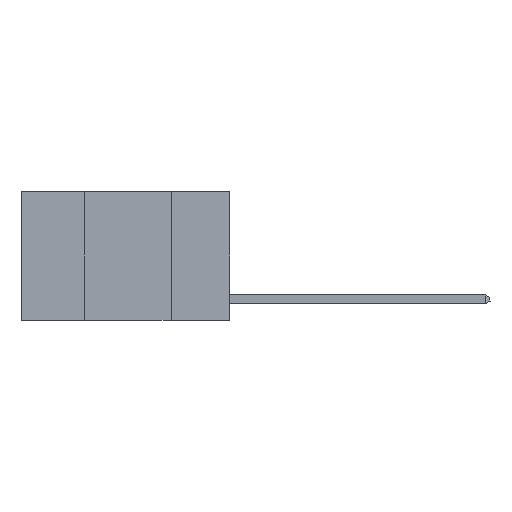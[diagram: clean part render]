
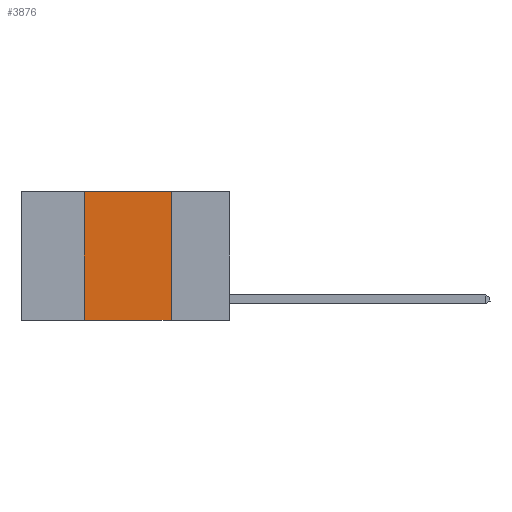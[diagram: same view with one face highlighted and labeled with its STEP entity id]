
A CAD part, left-side view. The second image highlights one B-rep face of the part: STEP entity #3876.
In plain terms, the highlighted planar face has unit normal (-1, 0, 0).
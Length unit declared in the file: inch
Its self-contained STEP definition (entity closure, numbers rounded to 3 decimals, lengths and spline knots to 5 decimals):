
#1446 = EDGE_CURVE ( 'NONE', #4142, #4504, #2782, .T. ) ;
#2782 = LINE ( 'NONE', #12712, #23775 ) ;
#3180 = AXIS2_PLACEMENT_3D ( 'NONE', #5985, #12367, #26948 ) ;
#3876 = ADVANCED_FACE ( 'NONE', ( #21820 ), #16523, .F. ) ;
#4142 = VERTEX_POINT ( 'NONE', #23662 ) ;
#4504 = VERTEX_POINT ( 'NONE', #22647 ) ;
#5744 = VECTOR ( 'NONE', #5981, 39.37008 ) ;
#5981 = DIRECTION ( 'NONE',  ( 0., -1., 0. ) ) ;
#5985 = CARTESIAN_POINT ( 'NONE',  ( 0., 0.6, 0. ) ) ;
#6893 = EDGE_CURVE ( 'NONE', #4504, #24385, #7233, .T. ) ;
#7233 = LINE ( 'NONE', #17156, #17783 ) ;
#7888 = CARTESIAN_POINT ( 'NONE',  ( 0., 0.17, -0.37 ) ) ;
#8192 = ORIENTED_EDGE ( 'NONE', *, *, #23771, .T. ) ;
#10487 = DIRECTION ( 'NONE',  ( 0., -1., 0. ) ) ;
#11844 = ORIENTED_EDGE ( 'NONE', *, *, #1446, .F. ) ;
#12367 = DIRECTION ( 'NONE',  ( 1., 0., 0. ) ) ;
#12712 = CARTESIAN_POINT ( 'NONE',  ( 0., 0.6, 0. ) ) ;
#14300 = CARTESIAN_POINT ( 'NONE',  ( 0., 0.42, 0. ) ) ;
#15680 = EDGE_CURVE ( 'NONE', #21870, #4142, #24409, .T. ) ;
#16521 = CARTESIAN_POINT ( 'NONE',  ( 0., 0.6, -0.37 ) ) ;
#16523 = PLANE ( 'NONE',  #3180 ) ;
#17156 = CARTESIAN_POINT ( 'NONE',  ( 0., 0.17, 0. ) ) ;
#17783 = VECTOR ( 'NONE', #19233, 39.37008 ) ;
#18492 = DIRECTION ( 'NONE',  ( 0., 0., 1. ) ) ;
#19233 = DIRECTION ( 'NONE',  ( 0., 0., -1. ) ) ;
#20219 = CARTESIAN_POINT ( 'NONE',  ( 0., 0.42, -0.37 ) ) ;
#21820 = FACE_OUTER_BOUND ( 'NONE', #22586, .T. ) ;
#21870 = VERTEX_POINT ( 'NONE', #20219 ) ;
#22305 = ORIENTED_EDGE ( 'NONE', *, *, #6893, .F. ) ;
#22486 = LINE ( 'NONE', #16521, #5744 ) ;
#22586 = EDGE_LOOP ( 'NONE', ( #22305, #11844, #24246, #8192 ) ) ;
#22647 = CARTESIAN_POINT ( 'NONE',  ( 0., 0.17, 0. ) ) ;
#23662 = CARTESIAN_POINT ( 'NONE',  ( 0., 0.42, 0. ) ) ;
#23771 = EDGE_CURVE ( 'NONE', #21870, #24385, #22486, .T. ) ;
#23775 = VECTOR ( 'NONE', #10487, 39.37008 ) ;
#23777 = VECTOR ( 'NONE', #18492, 39.37008 ) ;
#24246 = ORIENTED_EDGE ( 'NONE', *, *, #15680, .F. ) ;
#24385 = VERTEX_POINT ( 'NONE', #7888 ) ;
#24409 = LINE ( 'NONE', #14300, #23777 ) ;
#26948 = DIRECTION ( 'NONE',  ( 0., 0., -1. ) ) ;
